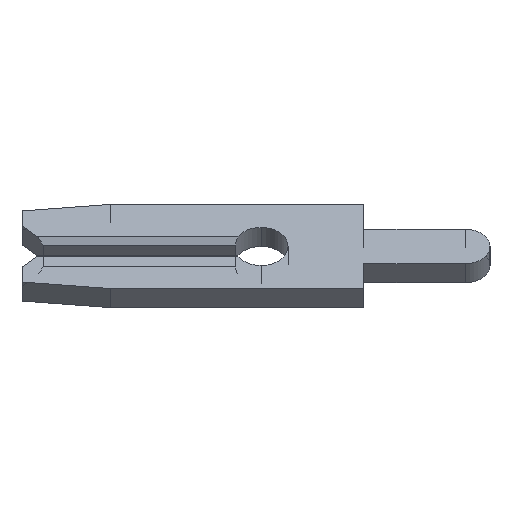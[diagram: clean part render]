
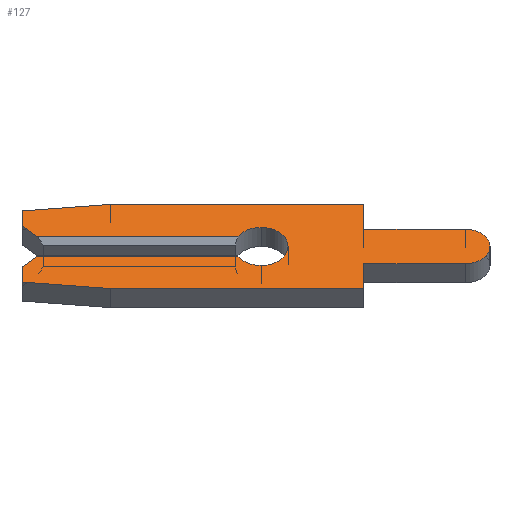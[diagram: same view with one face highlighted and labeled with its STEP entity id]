
A CAD part, left-side view. The second image highlights one B-rep face of the part: STEP entity #127.
In plain terms, the highlighted face is planar.
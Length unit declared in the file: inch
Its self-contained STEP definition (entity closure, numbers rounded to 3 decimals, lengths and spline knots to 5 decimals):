
#2 = EDGE_CURVE ( 'NONE', #385, #261, #539, .T. ) ;
#11 = VERTEX_POINT ( 'NONE', #1115 ) ;
#41 = VECTOR ( 'NONE', #2075, 39.37008 ) ;
#51 = EDGE_CURVE ( 'NONE', #2378, #232, #1235, .T. ) ;
#52 = DIRECTION ( 'NONE',  ( 0., 0., -1. ) ) ;
#68 = ORIENTED_EDGE ( 'NONE', *, *, #2165, .F. ) ;
#77 = CARTESIAN_POINT ( 'NONE',  ( -0.013, 0.216, -0.013 ) ) ;
#94 = VECTOR ( 'NONE', #502, 39.37008 ) ;
#95 = CARTESIAN_POINT ( 'NONE',  ( -0.013, 0., 0. ) ) ;
#96 = ORIENTED_EDGE ( 'NONE', *, *, #130, .F. ) ;
#126 = LINE ( 'NONE', #301, #2049 ) ;
#127 = ADVANCED_FACE ( 'NONE', ( #737 ), #1341, .F. ) ;
#130 = EDGE_CURVE ( 'NONE', #2318, #1585, #677, .T. ) ;
#134 = VECTOR ( 'NONE', #388, 39.37008 ) ;
#155 = EDGE_CURVE ( 'NONE', #2378, #261, #1851, .T. ) ;
#178 = ORIENTED_EDGE ( 'NONE', *, *, #691, .F. ) ;
#206 = LINE ( 'NONE', #1614, #2133 ) ;
#208 = ORIENTED_EDGE ( 'NONE', *, *, #663, .F. ) ;
#232 = VERTEX_POINT ( 'NONE', #2306 ) ;
#245 = CARTESIAN_POINT ( 'NONE',  ( -0.013, 0., 0.026 ) ) ;
#261 = VERTEX_POINT ( 'NONE', #616 ) ;
#263 = ORIENTED_EDGE ( 'NONE', *, *, #2258, .F. ) ;
#278 = CARTESIAN_POINT ( 'NONE',  ( -0.013, -0.099, -0.0575 ) ) ;
#298 = ORIENTED_EDGE ( 'NONE', *, *, #2174, .F. ) ;
#301 = CARTESIAN_POINT ( 'NONE',  ( -0.013, 0.146, 0.0575 ) ) ;
#328 = EDGE_LOOP ( 'NONE', ( #1101, #1208, #538, #2161, #263, #1352, #1644, #1265, #68, #178, #298, #792, #96, #1734, #208, #1259, #855, #991 ) ) ;
#350 = DIRECTION ( 'NONE',  ( 1., 0., 0. ) ) ;
#351 = VECTOR ( 'NONE', #1811, 39.37008 ) ;
#353 = VECTOR ( 'NONE', #602, 39.37008 ) ;
#373 = CARTESIAN_POINT ( 'NONE',  ( -0.013, -0.1975, 0. ) ) ;
#377 = VECTOR ( 'NONE', #628, 39.37008 ) ;
#382 = VECTOR ( 'NONE', #1082, 39.37008 ) ;
#385 = VERTEX_POINT ( 'NONE', #245 ) ;
#388 = DIRECTION ( 'NONE',  ( 0., 0., -1. ) ) ;
#427 = DIRECTION ( 'NONE',  ( 1., 0., 0. ) ) ;
#465 = CARTESIAN_POINT ( 'NONE',  ( -0.013, 0.146, -0.0575 ) ) ;
#502 = DIRECTION ( 'NONE',  ( 0., 0., 1. ) ) ;
#507 = VECTOR ( 'NONE', #2118, 39.37008 ) ;
#529 = AXIS2_PLACEMENT_3D ( 'NONE', #966, #427, #52 ) ;
#535 = LINE ( 'NONE', #1059, #351 ) ;
#538 = ORIENTED_EDGE ( 'NONE', *, *, #586, .F. ) ;
#539 = CIRCLE ( 'NONE', #1694, 0.026 ) ;
#586 = EDGE_CURVE ( 'NONE', #1472, #385, #1994, .T. ) ;
#592 = DIRECTION ( 'NONE',  ( -1., 0., 0. ) ) ;
#602 = DIRECTION ( 'NONE',  ( 0., -0.707, 0.707 ) ) ;
#616 = CARTESIAN_POINT ( 'NONE',  ( -0.013, 0.02252, 0.013 ) ) ;
#622 = CARTESIAN_POINT ( 'NONE',  ( -0.013, -0.099, -0.0235 ) ) ;
#628 = DIRECTION ( 'NONE',  ( 0., 1., 0. ) ) ;
#663 = EDGE_CURVE ( 'NONE', #2051, #11, #126, .T. ) ;
#677 = LINE ( 'NONE', #1930, #1357 ) ;
#691 = EDGE_CURVE ( 'NONE', #1992, #2021, #2317, .T. ) ;
#707 = CARTESIAN_POINT ( 'NONE',  ( -0.013, 0., 0. ) ) ;
#737 = FACE_OUTER_BOUND ( 'NONE', #328, .T. ) ;
#752 = EDGE_CURVE ( 'NONE', #817, #2051, #206, .T. ) ;
#770 = VERTEX_POINT ( 'NONE', #1034 ) ;
#783 = CARTESIAN_POINT ( 'NONE',  ( -0.013, 0.231, -0.028 ) ) ;
#792 = ORIENTED_EDGE ( 'NONE', *, *, #1297, .F. ) ;
#793 = AXIS2_PLACEMENT_3D ( 'NONE', #707, #1620, #2015 ) ;
#814 = DIRECTION ( 'NONE',  ( 0., -1., 0. ) ) ;
#817 = VERTEX_POINT ( 'NONE', #862 ) ;
#844 = DIRECTION ( 'NONE',  ( 0., 0., -1. ) ) ;
#855 = ORIENTED_EDGE ( 'NONE', *, *, #883, .F. ) ;
#861 = VERTEX_POINT ( 'NONE', #1820 ) ;
#862 = CARTESIAN_POINT ( 'NONE',  ( -0.013, 0.231, 0.04857 ) ) ;
#883 = EDGE_CURVE ( 'NONE', #232, #817, #2076, .T. ) ;
#913 = EDGE_CURVE ( 'NONE', #861, #1848, #535, .T. ) ;
#939 = DIRECTION ( 'NONE',  ( 0., 0., -1. ) ) ;
#962 = LINE ( 'NONE', #1289, #382 ) ;
#966 = CARTESIAN_POINT ( 'NONE',  ( -0.013, 0., 0. ) ) ;
#970 = CARTESIAN_POINT ( 'NONE',  ( -0.013, -0.099, -0.0235 ) ) ;
#991 = ORIENTED_EDGE ( 'NONE', *, *, #51, .F. ) ;
#1017 = VECTOR ( 'NONE', #814, 39.37008 ) ;
#1034 = CARTESIAN_POINT ( 'NONE',  ( -0.013, -0.1975, -0.0235 ) ) ;
#1045 = DIRECTION ( 'NONE',  ( -1., 0., 0. ) ) ;
#1049 = LINE ( 'NONE', #2281, #134 ) ;
#1059 = CARTESIAN_POINT ( 'NONE',  ( -0.013, 0.231, -0.028 ) ) ;
#1082 = DIRECTION ( 'NONE',  ( 0., 0.995, 0.105 ) ) ;
#1101 = ORIENTED_EDGE ( 'NONE', *, *, #155, .T. ) ;
#1115 = CARTESIAN_POINT ( 'NONE',  ( -0.013, -0.099, 0.0575 ) ) ;
#1138 = CIRCLE ( 'NONE', #793, 0.026 ) ;
#1188 = DIRECTION ( 'NONE',  ( 0., -1., 0. ) ) ;
#1191 = EDGE_CURVE ( 'NONE', #1705, #1472, #1138, .T. ) ;
#1208 = ORIENTED_EDGE ( 'NONE', *, *, #2, .F. ) ;
#1235 = LINE ( 'NONE', #2247, #41 ) ;
#1259 = ORIENTED_EDGE ( 'NONE', *, *, #752, .F. ) ;
#1265 = ORIENTED_EDGE ( 'NONE', *, *, #1270, .F. ) ;
#1270 = EDGE_CURVE ( 'NONE', #2048, #861, #962, .T. ) ;
#1289 = CARTESIAN_POINT ( 'NONE',  ( -0.013, 0.231, -0.04857 ) ) ;
#1297 = EDGE_CURVE ( 'NONE', #1585, #770, #1466, .T. ) ;
#1304 = DIRECTION ( 'NONE',  ( 0., 0., 1. ) ) ;
#1338 = LINE ( 'NONE', #622, #507 ) ;
#1341 = PLANE ( 'NONE',  #529 ) ;
#1352 = ORIENTED_EDGE ( 'NONE', *, *, #2035, .F. ) ;
#1356 = CARTESIAN_POINT ( 'NONE',  ( -0.013, 0.146, -0.0575 ) ) ;
#1357 = VECTOR ( 'NONE', #1188, 39.37008 ) ;
#1360 = DIRECTION ( 'NONE',  ( 0., -1., 0. ) ) ;
#1377 = LINE ( 'NONE', #465, #377 ) ;
#1384 = CARTESIAN_POINT ( 'NONE',  ( -0.013, 0.216, 0.013 ) ) ;
#1390 = AXIS2_PLACEMENT_3D ( 'NONE', #95, #1045, #844 ) ;
#1393 = CARTESIAN_POINT ( 'NONE',  ( -0.013, 0., -0.013 ) ) ;
#1466 = CIRCLE ( 'NONE', #1623, 0.0235 ) ;
#1472 = VERTEX_POINT ( 'NONE', #1838 ) ;
#1536 = CARTESIAN_POINT ( 'NONE',  ( -0.013, 0., 0. ) ) ;
#1585 = VERTEX_POINT ( 'NONE', #1864 ) ;
#1614 = CARTESIAN_POINT ( 'NONE',  ( -0.013, 0.231, 0.04857 ) ) ;
#1620 = DIRECTION ( 'NONE',  ( -1., 0., 0. ) ) ;
#1623 = AXIS2_PLACEMENT_3D ( 'NONE', #373, #350, #1304 ) ;
#1644 = ORIENTED_EDGE ( 'NONE', *, *, #913, .F. ) ;
#1688 = CARTESIAN_POINT ( 'NONE',  ( -0.013, 0.146, 0.0575 ) ) ;
#1694 = AXIS2_PLACEMENT_3D ( 'NONE', #1536, #592, #939 ) ;
#1705 = VERTEX_POINT ( 'NONE', #1884 ) ;
#1728 = CARTESIAN_POINT ( 'NONE',  ( -0.013, 0.2105, -0.0075 ) ) ;
#1730 = CARTESIAN_POINT ( 'NONE',  ( -0.013, 0.231, 0.013 ) ) ;
#1734 = ORIENTED_EDGE ( 'NONE', *, *, #2003, .F. ) ;
#1797 = DIRECTION ( 'NONE',  ( 0., 0., -1. ) ) ;
#1811 = DIRECTION ( 'NONE',  ( 0., 0., 1. ) ) ;
#1820 = CARTESIAN_POINT ( 'NONE',  ( -0.013, 0.231, -0.04857 ) ) ;
#1838 = CARTESIAN_POINT ( 'NONE',  ( -0.013, 0., -0.026 ) ) ;
#1848 = VERTEX_POINT ( 'NONE', #783 ) ;
#1851 = LINE ( 'NONE', #1730, #2109 ) ;
#1864 = CARTESIAN_POINT ( 'NONE',  ( -0.013, -0.1975, 0.0235 ) ) ;
#1872 = LINE ( 'NONE', #1393, #1017 ) ;
#1884 = CARTESIAN_POINT ( 'NONE',  ( -0.013, 0.02252, -0.013 ) ) ;
#1930 = CARTESIAN_POINT ( 'NONE',  ( -0.013, -0.099, 0.0235 ) ) ;
#1992 = VERTEX_POINT ( 'NONE', #970 ) ;
#1994 = CIRCLE ( 'NONE', #1390, 0.026 ) ;
#2003 = EDGE_CURVE ( 'NONE', #11, #2318, #1049, .T. ) ;
#2015 = DIRECTION ( 'NONE',  ( 0., 0., -1. ) ) ;
#2021 = VERTEX_POINT ( 'NONE', #2085 ) ;
#2035 = EDGE_CURVE ( 'NONE', #1848, #2370, #2379, .T. ) ;
#2048 = VERTEX_POINT ( 'NONE', #1356 ) ;
#2049 = VECTOR ( 'NONE', #2341, 39.37008 ) ;
#2051 = VERTEX_POINT ( 'NONE', #1688 ) ;
#2075 = DIRECTION ( 'NONE',  ( 0., 0.707, 0.707 ) ) ;
#2076 = LINE ( 'NONE', #2203, #94 ) ;
#2085 = CARTESIAN_POINT ( 'NONE',  ( -0.013, -0.099, -0.0575 ) ) ;
#2108 = CARTESIAN_POINT ( 'NONE',  ( -0.013, -0.099, 0.0235 ) ) ;
#2109 = VECTOR ( 'NONE', #1360, 39.37008 ) ;
#2118 = DIRECTION ( 'NONE',  ( 0., 1., 0. ) ) ;
#2133 = VECTOR ( 'NONE', #2139, 39.37008 ) ;
#2139 = DIRECTION ( 'NONE',  ( 0., -0.995, 0.105 ) ) ;
#2161 = ORIENTED_EDGE ( 'NONE', *, *, #1191, .F. ) ;
#2165 = EDGE_CURVE ( 'NONE', #2021, #2048, #1377, .T. ) ;
#2174 = EDGE_CURVE ( 'NONE', #770, #1992, #1338, .T. ) ;
#2203 = CARTESIAN_POINT ( 'NONE',  ( -0.013, 0.231, 0.028 ) ) ;
#2247 = CARTESIAN_POINT ( 'NONE',  ( -0.013, 0.2105, 0.0075 ) ) ;
#2258 = EDGE_CURVE ( 'NONE', #2370, #1705, #1872, .T. ) ;
#2281 = CARTESIAN_POINT ( 'NONE',  ( -0.013, -0.099, 0.0575 ) ) ;
#2306 = CARTESIAN_POINT ( 'NONE',  ( -0.013, 0.231, 0.028 ) ) ;
#2317 = LINE ( 'NONE', #278, #2353 ) ;
#2318 = VERTEX_POINT ( 'NONE', #2108 ) ;
#2341 = DIRECTION ( 'NONE',  ( 0., -1., 0. ) ) ;
#2353 = VECTOR ( 'NONE', #1797, 39.37008 ) ;
#2370 = VERTEX_POINT ( 'NONE', #77 ) ;
#2378 = VERTEX_POINT ( 'NONE', #1384 ) ;
#2379 = LINE ( 'NONE', #1728, #353 ) ;
